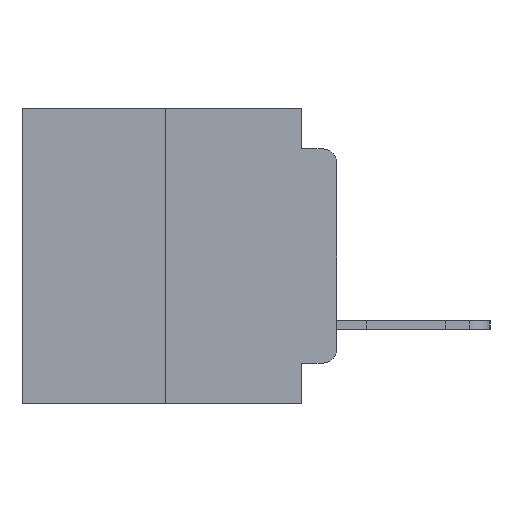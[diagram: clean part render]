
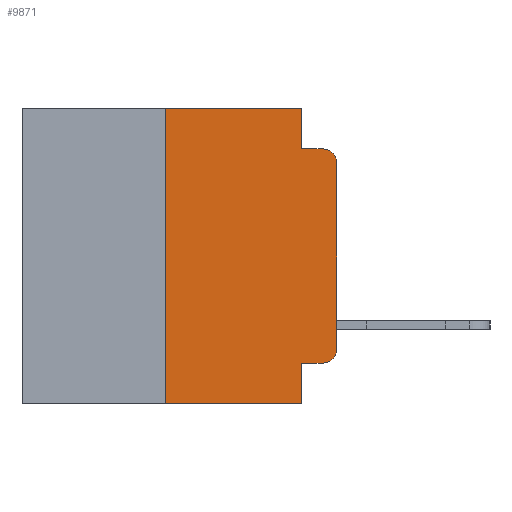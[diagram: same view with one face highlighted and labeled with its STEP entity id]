
A CAD part, left-side view. The second image highlights one B-rep face of the part: STEP entity #9871.
In plain terms, the highlighted planar face has unit normal (-1, 0, 0).
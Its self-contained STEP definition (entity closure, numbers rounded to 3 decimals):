
#451 = CARTESIAN_POINT ( 'NONE',  ( -75.603, 0., -3.467 ) ) ;
#679 = CIRCLE ( 'NONE', #21749, 0.508 ) ;
#811 = ORIENTED_EDGE ( 'NONE', *, *, #9089, .T. ) ;
#1829 = ORIENTED_EDGE ( 'NONE', *, *, #9383, .F. ) ;
#1910 = FACE_OUTER_BOUND ( 'NONE', #14922, .T. ) ;
#2426 = CARTESIAN_POINT ( 'NONE',  ( -75.603, 11.684, -5.486 ) ) ;
#2718 = ORIENTED_EDGE ( 'NONE', *, *, #22710, .F. ) ;
#2946 = VERTEX_POINT ( 'NONE', #451 ) ;
#3015 = DIRECTION ( 'NONE',  ( 0., -1., 0. ) ) ;
#3236 = LINE ( 'NONE', #4985, #9730 ) ;
#3445 = DIRECTION ( 'NONE',  ( 1., 0., 0. ) ) ;
#3677 = ORIENTED_EDGE ( 'NONE', *, *, #10563, .F. ) ;
#3852 = CARTESIAN_POINT ( 'NONE',  ( -75.603, 11.684, 5.486 ) ) ;
#4555 = EDGE_CURVE ( 'NONE', #17892, #2946, #15647, .T. ) ;
#4664 = VERTEX_POINT ( 'NONE', #21725 ) ;
#4985 = CARTESIAN_POINT ( 'NONE',  ( -75.603, 6.35, -5.486 ) ) ;
#6079 = ORIENTED_EDGE ( 'NONE', *, *, #4555, .T. ) ;
#6272 = VERTEX_POINT ( 'NONE', #17229 ) ;
#6634 = LINE ( 'NONE', #23320, #25836 ) ;
#7154 = VECTOR ( 'NONE', #17720, 1000. ) ;
#7400 = LINE ( 'NONE', #26357, #16661 ) ;
#7496 = ORIENTED_EDGE ( 'NONE', *, *, #10389, .F. ) ;
#7595 = EDGE_CURVE ( 'NONE', #26510, #4664, #26027, .T. ) ;
#7919 = EDGE_CURVE ( 'NONE', #9323, #10498, #679, .T. ) ;
#8407 = DIRECTION ( 'NONE',  ( 0., 0., -1. ) ) ;
#9089 = EDGE_CURVE ( 'NONE', #15629, #17892, #26618, .T. ) ;
#9323 = VERTEX_POINT ( 'NONE', #10146 ) ;
#9383 = EDGE_CURVE ( 'NONE', #11009, #6272, #23165, .T. ) ;
#9486 = CARTESIAN_POINT ( 'NONE',  ( -75.603, 6.35, 5.486 ) ) ;
#9730 = VECTOR ( 'NONE', #24807, 1000. ) ;
#9871 = ADVANCED_FACE ( 'NONE', ( #1910 ), #18471, .F. ) ;
#10146 = CARTESIAN_POINT ( 'NONE',  ( -75.603, 0., 3.467 ) ) ;
#10389 = EDGE_CURVE ( 'NONE', #13858, #10498, #24454, .T. ) ;
#10498 = VERTEX_POINT ( 'NONE', #23127 ) ;
#10530 = DIRECTION ( 'NONE',  ( 0., -1., 0. ) ) ;
#10563 = EDGE_CURVE ( 'NONE', #6272, #13858, #6634, .T. ) ;
#11009 = VERTEX_POINT ( 'NONE', #9486 ) ;
#11432 = CARTESIAN_POINT ( 'NONE',  ( -75.603, 1.295, 3.975 ) ) ;
#12038 = AXIS2_PLACEMENT_3D ( 'NONE', #12128, #3445, #18742 ) ;
#12128 = CARTESIAN_POINT ( 'NONE',  ( -75.603, 11.684, 5.486 ) ) ;
#12598 = ORIENTED_EDGE ( 'NONE', *, *, #22013, .T. ) ;
#13154 = VECTOR ( 'NONE', #14009, 1000. ) ;
#13215 = DIRECTION ( 'NONE',  ( 0., 0., -1. ) ) ;
#13781 = CARTESIAN_POINT ( 'NONE',  ( -75.603, 1.295, 3.975 ) ) ;
#13858 = VERTEX_POINT ( 'NONE', #13781 ) ;
#14009 = DIRECTION ( 'NONE',  ( 0., -1., 0. ) ) ;
#14074 = CARTESIAN_POINT ( 'NONE',  ( -75.603, 1.295, -3.975 ) ) ;
#14135 = CARTESIAN_POINT ( 'NONE',  ( -75.603, 1.295, -3.975 ) ) ;
#14426 = ORIENTED_EDGE ( 'NONE', *, *, #26803, .F. ) ;
#14922 = EDGE_LOOP ( 'NONE', ( #811, #6079, #12598, #18225, #7496, #3677, #1829, #2718, #17961, #14426 ) ) ;
#15629 = VERTEX_POINT ( 'NONE', #14135 ) ;
#15647 = CIRCLE ( 'NONE', #24600, 0.508 ) ;
#15978 = VECTOR ( 'NONE', #3015, 1000. ) ;
#16661 = VECTOR ( 'NONE', #13215, 1000. ) ;
#16671 = CARTESIAN_POINT ( 'NONE',  ( -75.603, 6.35, -5.486 ) ) ;
#17229 = CARTESIAN_POINT ( 'NONE',  ( -75.603, 1.295, 5.486 ) ) ;
#17720 = DIRECTION ( 'NONE',  ( 0., -1., 0. ) ) ;
#17892 = VERTEX_POINT ( 'NONE', #27833 ) ;
#17961 = ORIENTED_EDGE ( 'NONE', *, *, #7595, .T. ) ;
#18225 = ORIENTED_EDGE ( 'NONE', *, *, #7919, .T. ) ;
#18229 = DIRECTION ( 'NONE',  ( 0., 0., 1. ) ) ;
#18471 = PLANE ( 'NONE',  #12038 ) ;
#18742 = DIRECTION ( 'NONE',  ( 0., 0., -1. ) ) ;
#19785 = CARTESIAN_POINT ( 'NONE',  ( -75.603, 0., 5.486 ) ) ;
#20603 = CARTESIAN_POINT ( 'NONE',  ( -75.603, 0.508, -3.467 ) ) ;
#20773 = LINE ( 'NONE', #19785, #28329 ) ;
#21561 = CARTESIAN_POINT ( 'NONE',  ( -75.603, 0.508, 3.467 ) ) ;
#21725 = CARTESIAN_POINT ( 'NONE',  ( -75.603, 1.295, -5.486 ) ) ;
#21749 = AXIS2_PLACEMENT_3D ( 'NONE', #21561, #25365, #8407 ) ;
#22013 = EDGE_CURVE ( 'NONE', #2946, #9323, #20773, .T. ) ;
#22710 = EDGE_CURVE ( 'NONE', #26510, #11009, #3236, .T. ) ;
#22795 = DIRECTION ( 'NONE',  ( -1., 0., 0. ) ) ;
#23127 = CARTESIAN_POINT ( 'NONE',  ( -75.603, 0.508, 3.975 ) ) ;
#23165 = LINE ( 'NONE', #3852, #27639 ) ;
#23320 = CARTESIAN_POINT ( 'NONE',  ( -75.603, 1.295, 0. ) ) ;
#24454 = LINE ( 'NONE', #11432, #13154 ) ;
#24600 = AXIS2_PLACEMENT_3D ( 'NONE', #20603, #22795, #24994 ) ;
#24807 = DIRECTION ( 'NONE',  ( 0., 0., 1. ) ) ;
#24994 = DIRECTION ( 'NONE',  ( 0., 0., -1. ) ) ;
#25365 = DIRECTION ( 'NONE',  ( -1., 0., 0. ) ) ;
#25614 = DIRECTION ( 'NONE',  ( 0., 0., -1. ) ) ;
#25836 = VECTOR ( 'NONE', #25614, 1000. ) ;
#26027 = LINE ( 'NONE', #2426, #7154 ) ;
#26357 = CARTESIAN_POINT ( 'NONE',  ( -75.603, 1.295, 0. ) ) ;
#26510 = VERTEX_POINT ( 'NONE', #16671 ) ;
#26618 = LINE ( 'NONE', #14074, #15978 ) ;
#26803 = EDGE_CURVE ( 'NONE', #15629, #4664, #7400, .T. ) ;
#27639 = VECTOR ( 'NONE', #10530, 1000. ) ;
#27833 = CARTESIAN_POINT ( 'NONE',  ( -75.603, 0.508, -3.975 ) ) ;
#28329 = VECTOR ( 'NONE', #18229, 1000. ) ;
